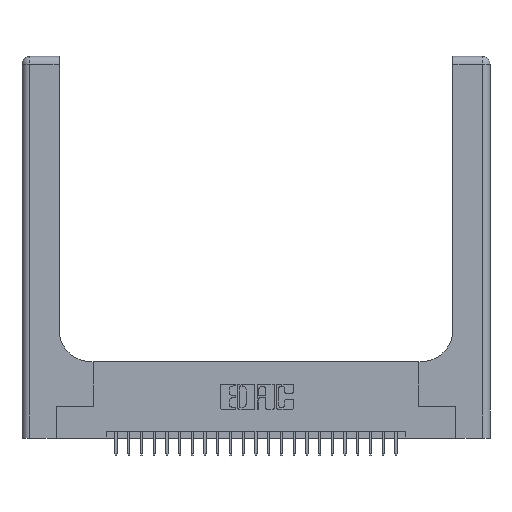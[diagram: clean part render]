
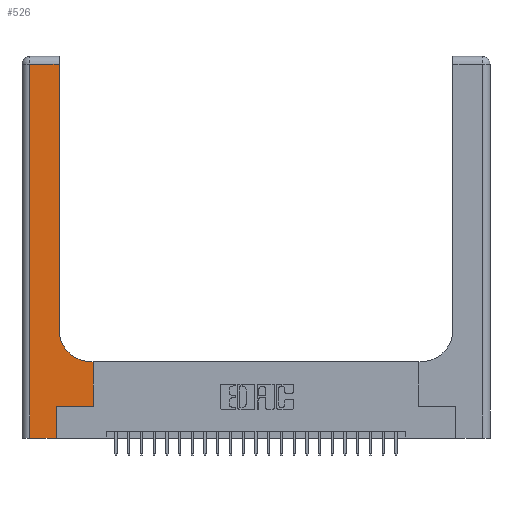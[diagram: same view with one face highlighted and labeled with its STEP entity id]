
A CAD part, top view. The second image highlights one B-rep face of the part: STEP entity #526.
In plain terms, the highlighted planar face has unit normal (0, 0, 1).
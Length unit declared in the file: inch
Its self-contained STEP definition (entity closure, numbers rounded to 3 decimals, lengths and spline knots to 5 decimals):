
#496 = CARTESIAN_POINT ( 'NONE',  ( 0.2915, 3., 0.37 ) ) ;
#526 = ADVANCED_FACE ( 'NONE', ( #3044 ), #12975, .F. ) ;
#651 = DIRECTION ( 'NONE',  ( 0., 1., 0. ) ) ;
#1135 = CIRCLE ( 'NONE', #19549, 0.25 ) ;
#1487 = VECTOR ( 'NONE', #13943, 39.37008 ) ;
#1559 = CARTESIAN_POINT ( 'NONE',  ( 0.5415, 0.85, 0.37 ) ) ;
#1876 = EDGE_CURVE ( 'NONE', #8582, #23914, #19671, .T. ) ;
#2208 = VECTOR ( 'NONE', #18204, 39.37008 ) ;
#3044 = FACE_OUTER_BOUND ( 'NONE', #3799, .T. ) ;
#3047 = CARTESIAN_POINT ( 'NONE',  ( 0.5585, 0.25, 0.37 ) ) ;
#3101 = AXIS2_PLACEMENT_3D ( 'NONE', #12849, #18755, #15205 ) ;
#3512 = CARTESIAN_POINT ( 'NONE',  ( 0.06, 0., 0.37 ) ) ;
#3685 = EDGE_CURVE ( 'NONE', #10985, #8582, #4960, .T. ) ;
#3799 = EDGE_LOOP ( 'NONE', ( #15176, #21505, #10525, #8798, #19713, #11422, #17110, #9210, #18581 ) ) ;
#4286 = EDGE_CURVE ( 'NONE', #14208, #9665, #23996, .T. ) ;
#4305 = CARTESIAN_POINT ( 'NONE',  ( 0.269, 0., 0.37 ) ) ;
#4938 = VERTEX_POINT ( 'NONE', #24556 ) ;
#4960 = LINE ( 'NONE', #11090, #11907 ) ;
#5022 = DIRECTION ( 'NONE',  ( 1., 0., 0. ) ) ;
#5976 = CARTESIAN_POINT ( 'NONE',  ( 0.5585, 0.25, 0.37 ) ) ;
#6032 = EDGE_CURVE ( 'NONE', #9665, #24557, #1135, .T. ) ;
#8376 = CARTESIAN_POINT ( 'NONE',  ( 0.5415, 0.6, 0.37 ) ) ;
#8582 = VERTEX_POINT ( 'NONE', #21146 ) ;
#8758 = VECTOR ( 'NONE', #651, 39.37008 ) ;
#8798 = ORIENTED_EDGE ( 'NONE', *, *, #14475, .T. ) ;
#9210 = ORIENTED_EDGE ( 'NONE', *, *, #4286, .T. ) ;
#9259 = CARTESIAN_POINT ( 'NONE',  ( 0.2915, 0.85, 0.37 ) ) ;
#9665 = VERTEX_POINT ( 'NONE', #8376 ) ;
#9681 = DIRECTION ( 'NONE',  ( 0., -1., 0. ) ) ;
#10525 = ORIENTED_EDGE ( 'NONE', *, *, #1876, .T. ) ;
#10985 = VERTEX_POINT ( 'NONE', #18112 ) ;
#11090 = CARTESIAN_POINT ( 'NONE',  ( 0., 2.94, 0.37 ) ) ;
#11420 = VECTOR ( 'NONE', #9681, 39.37008 ) ;
#11422 = ORIENTED_EDGE ( 'NONE', *, *, #15908, .T. ) ;
#11750 = EDGE_CURVE ( 'NONE', #24557, #10985, #20431, .T. ) ;
#11907 = VECTOR ( 'NONE', #22913, 39.37008 ) ;
#12405 = DIRECTION ( 'NONE',  ( 0., 1., 0. ) ) ;
#12849 = CARTESIAN_POINT ( 'NONE',  ( 0., 3., 0.37 ) ) ;
#12975 = PLANE ( 'NONE',  #3101 ) ;
#13186 = EDGE_CURVE ( 'NONE', #16671, #4938, #18728, .T. ) ;
#13943 = DIRECTION ( 'NONE',  ( 0., 1., 0. ) ) ;
#14208 = VERTEX_POINT ( 'NONE', #14991 ) ;
#14422 = CARTESIAN_POINT ( 'NONE',  ( 0.2915, 0.6, 0.37 ) ) ;
#14475 = EDGE_CURVE ( 'NONE', #23914, #16671, #25073, .T. ) ;
#14991 = CARTESIAN_POINT ( 'NONE',  ( 0.5585, 0.6, 0.37 ) ) ;
#15176 = ORIENTED_EDGE ( 'NONE', *, *, #11750, .T. ) ;
#15205 = DIRECTION ( 'NONE',  ( -1., 0., 0. ) ) ;
#15219 = CARTESIAN_POINT ( 'NONE',  ( 0., 0., 0.37 ) ) ;
#15908 = EDGE_CURVE ( 'NONE', #4938, #20518, #20068, .T. ) ;
#16120 = DIRECTION ( 'NONE',  ( -1., 0., 0. ) ) ;
#16545 = VECTOR ( 'NONE', #16120, 39.37008 ) ;
#16671 = VERTEX_POINT ( 'NONE', #4305 ) ;
#17110 = ORIENTED_EDGE ( 'NONE', *, *, #18058, .T. ) ;
#17172 = LINE ( 'NONE', #5976, #1487 ) ;
#17261 = DIRECTION ( 'NONE',  ( 0., 0., -1. ) ) ;
#17588 = VECTOR ( 'NONE', #12405, 39.37008 ) ;
#17942 = CARTESIAN_POINT ( 'NONE',  ( 0.06, 3., 0.37 ) ) ;
#18058 = EDGE_CURVE ( 'NONE', #20518, #14208, #17172, .T. ) ;
#18112 = CARTESIAN_POINT ( 'NONE',  ( 0.2915, 2.94, 0.37 ) ) ;
#18204 = DIRECTION ( 'NONE',  ( 1., 0., 0. ) ) ;
#18581 = ORIENTED_EDGE ( 'NONE', *, *, #6032, .T. ) ;
#18728 = LINE ( 'NONE', #22058, #8758 ) ;
#18755 = DIRECTION ( 'NONE',  ( 0., 0., -1. ) ) ;
#19372 = DIRECTION ( 'NONE',  ( 1., 0., 0. ) ) ;
#19549 = AXIS2_PLACEMENT_3D ( 'NONE', #1559, #17261, #19372 ) ;
#19671 = LINE ( 'NONE', #17942, #11420 ) ;
#19713 = ORIENTED_EDGE ( 'NONE', *, *, #13186, .T. ) ;
#20068 = LINE ( 'NONE', #20591, #2208 ) ;
#20431 = LINE ( 'NONE', #496, #17588 ) ;
#20518 = VERTEX_POINT ( 'NONE', #3047 ) ;
#20591 = CARTESIAN_POINT ( 'NONE',  ( 0.269, 0.25, 0.37 ) ) ;
#21146 = CARTESIAN_POINT ( 'NONE',  ( 0.06, 2.94, 0.37 ) ) ;
#21505 = ORIENTED_EDGE ( 'NONE', *, *, #3685, .T. ) ;
#22058 = CARTESIAN_POINT ( 'NONE',  ( 0.269, 0., 0.37 ) ) ;
#22913 = DIRECTION ( 'NONE',  ( -1., 0., 0. ) ) ;
#23914 = VERTEX_POINT ( 'NONE', #3512 ) ;
#23996 = LINE ( 'NONE', #14422, #16545 ) ;
#24556 = CARTESIAN_POINT ( 'NONE',  ( 0.269, 0.25, 0.37 ) ) ;
#24557 = VERTEX_POINT ( 'NONE', #9259 ) ;
#25073 = LINE ( 'NONE', #15219, #25614 ) ;
#25614 = VECTOR ( 'NONE', #5022, 39.37008 ) ;
